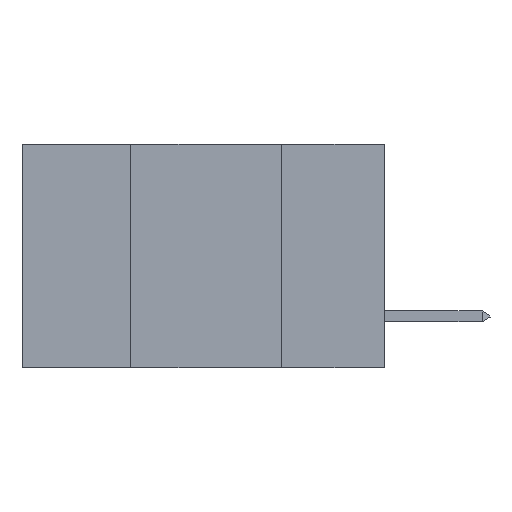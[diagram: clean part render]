
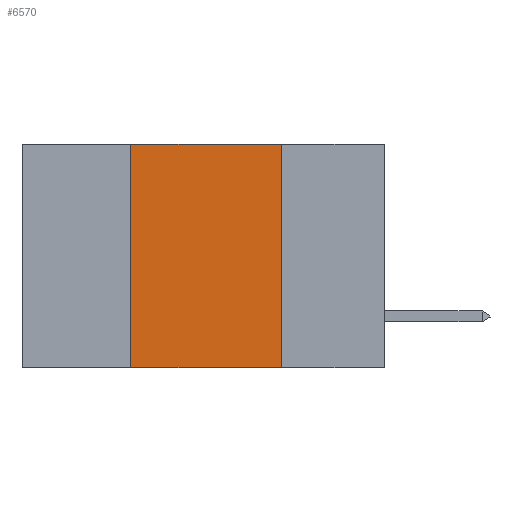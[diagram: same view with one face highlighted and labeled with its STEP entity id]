
A CAD part, left-side view. The second image highlights one B-rep face of the part: STEP entity #6570.
In plain terms, the highlighted planar face has unit normal (-1, 0, 0).
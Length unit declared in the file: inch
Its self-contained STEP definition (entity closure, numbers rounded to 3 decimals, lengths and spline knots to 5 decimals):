
#165 = VERTEX_POINT ( 'NONE', #25101 ) ;
#840 = CARTESIAN_POINT ( 'NONE',  ( 0., 0.6, 0. ) ) ;
#2458 = PLANE ( 'NONE',  #3319 ) ;
#2924 = EDGE_CURVE ( 'NONE', #16050, #29729, #5742, .T. ) ;
#3319 = AXIS2_PLACEMENT_3D ( 'NONE', #5488, #20216, #9131 ) ;
#3608 = LINE ( 'NONE', #23106, #24905 ) ;
#4313 = VECTOR ( 'NONE', #25869, 39.37008 ) ;
#4637 = ORIENTED_EDGE ( 'NONE', *, *, #2924, .T. ) ;
#4866 = DIRECTION ( 'NONE',  ( 0., 0., -1. ) ) ;
#4948 = VECTOR ( 'NONE', #14928, 39.37008 ) ;
#5488 = CARTESIAN_POINT ( 'NONE',  ( 0., 0.6, 0. ) ) ;
#5742 = LINE ( 'NONE', #16485, #4313 ) ;
#6570 = ADVANCED_FACE ( 'NONE', ( #18261 ), #2458, .F. ) ;
#9131 = DIRECTION ( 'NONE',  ( 0., 0., -1. ) ) ;
#9616 = CARTESIAN_POINT ( 'NONE',  ( 0., 0.17, 0. ) ) ;
#9846 = EDGE_CURVE ( 'NONE', #16050, #15804, #3608, .T. ) ;
#13526 = LINE ( 'NONE', #9616, #16716 ) ;
#13758 = EDGE_LOOP ( 'NONE', ( #23971, #24527, #26505, #4637 ) ) ;
#14928 = DIRECTION ( 'NONE',  ( 0., -1., 0. ) ) ;
#15458 = LINE ( 'NONE', #840, #4948 ) ;
#15804 = VERTEX_POINT ( 'NONE', #27318 ) ;
#16050 = VERTEX_POINT ( 'NONE', #26754 ) ;
#16485 = CARTESIAN_POINT ( 'NONE',  ( 0., 0.6, -0.37 ) ) ;
#16716 = VECTOR ( 'NONE', #4866, 39.37008 ) ;
#18261 = FACE_OUTER_BOUND ( 'NONE', #13758, .T. ) ;
#20216 = DIRECTION ( 'NONE',  ( 1., 0., 0. ) ) ;
#22839 = EDGE_CURVE ( 'NONE', #15804, #165, #15458, .T. ) ;
#23106 = CARTESIAN_POINT ( 'NONE',  ( 0., 0.42, 0. ) ) ;
#23971 = ORIENTED_EDGE ( 'NONE', *, *, #26173, .F. ) ;
#24527 = ORIENTED_EDGE ( 'NONE', *, *, #22839, .F. ) ;
#24905 = VECTOR ( 'NONE', #25785, 39.37008 ) ;
#25101 = CARTESIAN_POINT ( 'NONE',  ( 0., 0.17, 0. ) ) ;
#25785 = DIRECTION ( 'NONE',  ( 0., 0., 1. ) ) ;
#25869 = DIRECTION ( 'NONE',  ( 0., -1., 0. ) ) ;
#26173 = EDGE_CURVE ( 'NONE', #165, #29729, #13526, .T. ) ;
#26505 = ORIENTED_EDGE ( 'NONE', *, *, #9846, .F. ) ;
#26754 = CARTESIAN_POINT ( 'NONE',  ( 0., 0.42, -0.37 ) ) ;
#27147 = CARTESIAN_POINT ( 'NONE',  ( 0., 0.17, -0.37 ) ) ;
#27318 = CARTESIAN_POINT ( 'NONE',  ( 0., 0.42, 0. ) ) ;
#29729 = VERTEX_POINT ( 'NONE', #27147 ) ;
